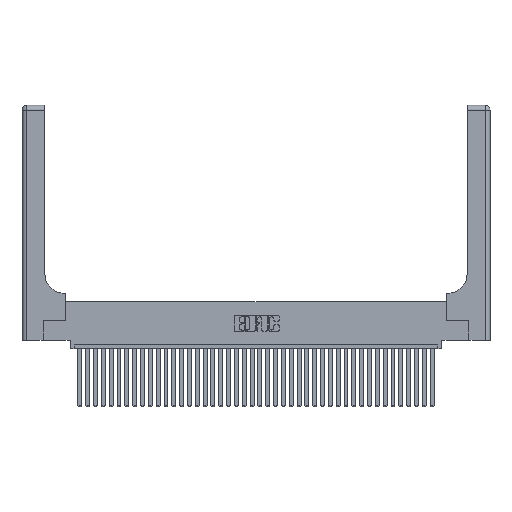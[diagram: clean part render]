
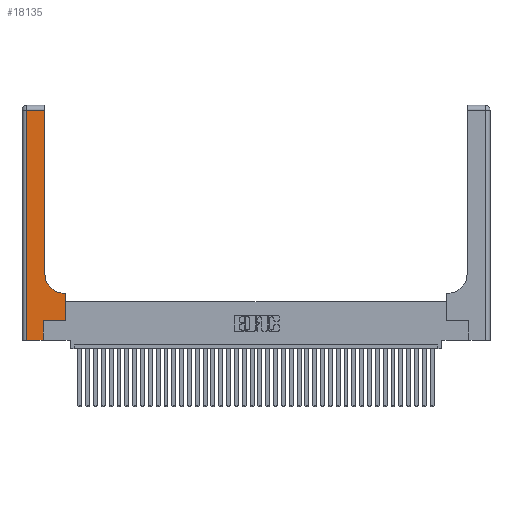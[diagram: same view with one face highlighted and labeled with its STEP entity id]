
A CAD part, top view. The second image highlights one B-rep face of the part: STEP entity #18135.
In plain terms, the highlighted planar face has unit normal (0, 0, 1).
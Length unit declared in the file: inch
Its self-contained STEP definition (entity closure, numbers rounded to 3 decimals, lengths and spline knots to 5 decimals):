
#31 = ORIENTED_EDGE ( 'NONE', *, *, #16494, .T. ) ;
#162 = CARTESIAN_POINT ( 'NONE',  ( 0., 0., 0.37 ) ) ;
#484 = EDGE_CURVE ( 'NONE', #7331, #29758, #33176, .T. ) ;
#625 = VERTEX_POINT ( 'NONE', #11831 ) ;
#948 = DIRECTION ( 'NONE',  ( -1., 0., 0. ) ) ;
#1506 = VECTOR ( 'NONE', #20863, 39.37008 ) ;
#1933 = EDGE_CURVE ( 'NONE', #17050, #38992, #18815, .T. ) ;
#3222 = CARTESIAN_POINT ( 'NONE',  ( 0., 2.94, 0.37 ) ) ;
#3540 = EDGE_CURVE ( 'NONE', #11875, #19556, #28943, .T. ) ;
#3599 = DIRECTION ( 'NONE',  ( 1., 0., 0. ) ) ;
#3685 = CARTESIAN_POINT ( 'NONE',  ( 0.06, 2.94, 0.37 ) ) ;
#4353 = LINE ( 'NONE', #30487, #1506 ) ;
#4750 = LINE ( 'NONE', #162, #6674 ) ;
#5937 = DIRECTION ( 'NONE',  ( 0., 1., 0. ) ) ;
#6556 = CARTESIAN_POINT ( 'NONE',  ( 0.5415, 0.85, 0.37 ) ) ;
#6674 = VECTOR ( 'NONE', #3599, 39.37008 ) ;
#7331 = VERTEX_POINT ( 'NONE', #27236 ) ;
#7655 = VERTEX_POINT ( 'NONE', #37835 ) ;
#8347 = CARTESIAN_POINT ( 'NONE',  ( 0.269, 0.25, 0.37 ) ) ;
#8366 = ORIENTED_EDGE ( 'NONE', *, *, #33205, .T. ) ;
#8520 = VECTOR ( 'NONE', #9823, 39.37008 ) ;
#9290 = DIRECTION ( 'NONE',  ( -1., 0., 0. ) ) ;
#9310 = CIRCLE ( 'NONE', #25170, 0.25 ) ;
#9728 = EDGE_LOOP ( 'NONE', ( #31, #11463, #18000, #21511, #11292, #31698, #29480, #8366, #19219 ) ) ;
#9823 = DIRECTION ( 'NONE',  ( -1., 0., 0. ) ) ;
#10312 = VECTOR ( 'NONE', #14539, 39.37008 ) ;
#10387 = FACE_OUTER_BOUND ( 'NONE', #9728, .T. ) ;
#10539 = CARTESIAN_POINT ( 'NONE',  ( 0.06, 0., 0.37 ) ) ;
#11292 = ORIENTED_EDGE ( 'NONE', *, *, #1933, .T. ) ;
#11463 = ORIENTED_EDGE ( 'NONE', *, *, #3540, .T. ) ;
#11612 = CARTESIAN_POINT ( 'NONE',  ( 0.269, 0., 0.37 ) ) ;
#11679 = EDGE_CURVE ( 'NONE', #19556, #14951, #4353, .T. ) ;
#11831 = CARTESIAN_POINT ( 'NONE',  ( 0.2915, 0.85, 0.37 ) ) ;
#11875 = VERTEX_POINT ( 'NONE', #15941 ) ;
#12207 = DIRECTION ( 'NONE',  ( 0., 0., -1. ) ) ;
#14213 = AXIS2_PLACEMENT_3D ( 'NONE', #15533, #12207, #9290 ) ;
#14539 = DIRECTION ( 'NONE',  ( 0., 1., 0. ) ) ;
#14951 = VERTEX_POINT ( 'NONE', #10539 ) ;
#15533 = CARTESIAN_POINT ( 'NONE',  ( 0., 3., 0.37 ) ) ;
#15941 = CARTESIAN_POINT ( 'NONE',  ( 0.2915, 2.94, 0.37 ) ) ;
#16322 = DIRECTION ( 'NONE',  ( 0., 1., 0. ) ) ;
#16494 = EDGE_CURVE ( 'NONE', #625, #11875, #33239, .T. ) ;
#17011 = DIRECTION ( 'NONE',  ( 1., 0., 0. ) ) ;
#17050 = VERTEX_POINT ( 'NONE', #27815 ) ;
#18000 = ORIENTED_EDGE ( 'NONE', *, *, #11679, .T. ) ;
#18114 = CARTESIAN_POINT ( 'NONE',  ( 0.5585, 0.25, 0.37 ) ) ;
#18135 = ADVANCED_FACE ( 'NONE', ( #10387 ), #36553, .F. ) ;
#18331 = DIRECTION ( 'NONE',  ( 1., 0., 0. ) ) ;
#18580 = VECTOR ( 'NONE', #16322, 39.37008 ) ;
#18815 = LINE ( 'NONE', #11612, #10312 ) ;
#19053 = VECTOR ( 'NONE', #948, 39.37008 ) ;
#19219 = ORIENTED_EDGE ( 'NONE', *, *, #19995, .T. ) ;
#19556 = VERTEX_POINT ( 'NONE', #3685 ) ;
#19995 = EDGE_CURVE ( 'NONE', #7655, #625, #9310, .T. ) ;
#20366 = EDGE_CURVE ( 'NONE', #38992, #7331, #20658, .T. ) ;
#20658 = LINE ( 'NONE', #8347, #29650 ) ;
#20863 = DIRECTION ( 'NONE',  ( 0., -1., 0. ) ) ;
#21446 = LINE ( 'NONE', #31411, #19053 ) ;
#21511 = ORIENTED_EDGE ( 'NONE', *, *, #38001, .T. ) ;
#23241 = VECTOR ( 'NONE', #5937, 39.37008 ) ;
#24314 = DIRECTION ( 'NONE',  ( 0., 0., -1. ) ) ;
#25170 = AXIS2_PLACEMENT_3D ( 'NONE', #6556, #24314, #18331 ) ;
#27236 = CARTESIAN_POINT ( 'NONE',  ( 0.5585, 0.25, 0.37 ) ) ;
#27815 = CARTESIAN_POINT ( 'NONE',  ( 0.269, 0., 0.37 ) ) ;
#28943 = LINE ( 'NONE', #3222, #8520 ) ;
#29480 = ORIENTED_EDGE ( 'NONE', *, *, #484, .T. ) ;
#29650 = VECTOR ( 'NONE', #17011, 39.37008 ) ;
#29758 = VERTEX_POINT ( 'NONE', #38388 ) ;
#30487 = CARTESIAN_POINT ( 'NONE',  ( 0.06, 3., 0.37 ) ) ;
#31396 = CARTESIAN_POINT ( 'NONE',  ( 0.2915, 3., 0.37 ) ) ;
#31411 = CARTESIAN_POINT ( 'NONE',  ( 0.2915, 0.6, 0.37 ) ) ;
#31698 = ORIENTED_EDGE ( 'NONE', *, *, #20366, .T. ) ;
#33176 = LINE ( 'NONE', #18114, #23241 ) ;
#33205 = EDGE_CURVE ( 'NONE', #29758, #7655, #21446, .T. ) ;
#33239 = LINE ( 'NONE', #31396, #18580 ) ;
#35136 = CARTESIAN_POINT ( 'NONE',  ( 0.269, 0.25, 0.37 ) ) ;
#36553 = PLANE ( 'NONE',  #14213 ) ;
#37835 = CARTESIAN_POINT ( 'NONE',  ( 0.5415, 0.6, 0.37 ) ) ;
#38001 = EDGE_CURVE ( 'NONE', #14951, #17050, #4750, .T. ) ;
#38388 = CARTESIAN_POINT ( 'NONE',  ( 0.5585, 0.6, 0.37 ) ) ;
#38992 = VERTEX_POINT ( 'NONE', #35136 ) ;
